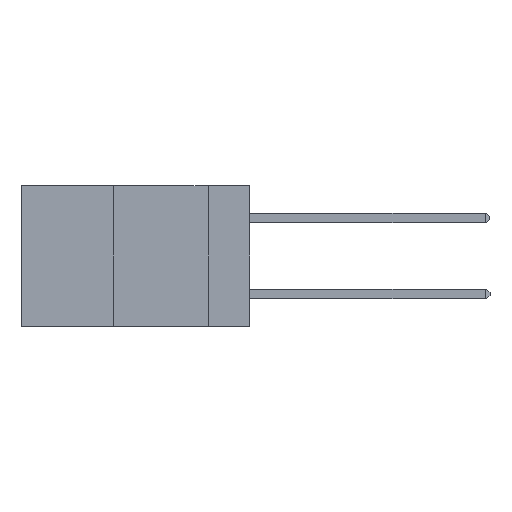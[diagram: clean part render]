
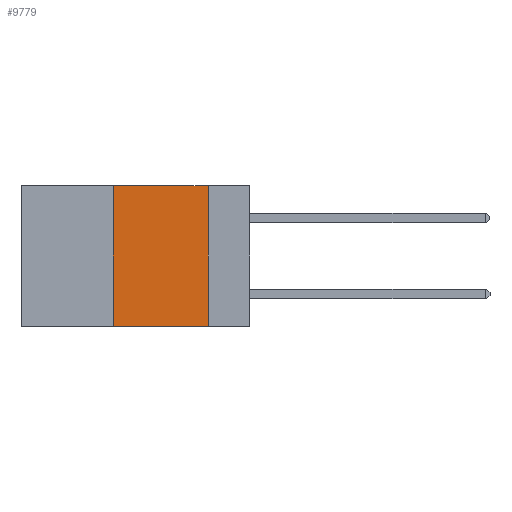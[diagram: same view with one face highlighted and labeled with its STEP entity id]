
A CAD part, left-side view. The second image highlights one B-rep face of the part: STEP entity #9779.
In plain terms, the highlighted planar face has unit normal (-1, 0, 0).
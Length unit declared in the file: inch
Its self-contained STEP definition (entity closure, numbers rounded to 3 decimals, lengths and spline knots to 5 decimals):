
#156 = CARTESIAN_POINT ( 'NONE',  ( 0., 0.6, 0. ) ) ;
#357 = DIRECTION ( 'NONE',  ( 0., 0., 1. ) ) ;
#439 = VERTEX_POINT ( 'NONE', #22396 ) ;
#813 = ORIENTED_EDGE ( 'NONE', *, *, #6139, .F. ) ;
#903 = EDGE_CURVE ( 'NONE', #3116, #18220, #6308, .T. ) ;
#1308 = CARTESIAN_POINT ( 'NONE',  ( 0., 0.6, 0. ) ) ;
#1581 = DIRECTION ( 'NONE',  ( 0., 0., -1. ) ) ;
#2209 = DIRECTION ( 'NONE',  ( 0., -1., 0. ) ) ;
#3116 = VERTEX_POINT ( 'NONE', #4890 ) ;
#4160 = DIRECTION ( 'NONE',  ( 0., -1., 0. ) ) ;
#4272 = FACE_OUTER_BOUND ( 'NONE', #5116, .T. ) ;
#4890 = CARTESIAN_POINT ( 'NONE',  ( 0., 0.36, -0.37 ) ) ;
#4979 = VECTOR ( 'NONE', #2209, 39.37008 ) ;
#5116 = EDGE_LOOP ( 'NONE', ( #8325, #813, #5667, #7925 ) ) ;
#5621 = VECTOR ( 'NONE', #1581, 39.37008 ) ;
#5667 = ORIENTED_EDGE ( 'NONE', *, *, #14387, .F. ) ;
#6139 = EDGE_CURVE ( 'NONE', #11145, #439, #9747, .T. ) ;
#6189 = LINE ( 'NONE', #10545, #5621 ) ;
#6308 = LINE ( 'NONE', #18498, #11646 ) ;
#6598 = LINE ( 'NONE', #20050, #20234 ) ;
#7240 = CARTESIAN_POINT ( 'NONE',  ( 0., 0.11, -0.37 ) ) ;
#7883 = AXIS2_PLACEMENT_3D ( 'NONE', #1308, #22674, #12191 ) ;
#7925 = ORIENTED_EDGE ( 'NONE', *, *, #903, .T. ) ;
#8325 = ORIENTED_EDGE ( 'NONE', *, *, #18668, .F. ) ;
#9747 = LINE ( 'NONE', #156, #4979 ) ;
#9779 = ADVANCED_FACE ( 'NONE', ( #4272 ), #20955, .F. ) ;
#10545 = CARTESIAN_POINT ( 'NONE',  ( 0., 0.11, 0. ) ) ;
#11145 = VERTEX_POINT ( 'NONE', #17614 ) ;
#11646 = VECTOR ( 'NONE', #4160, 39.37008 ) ;
#12191 = DIRECTION ( 'NONE',  ( 0., 0., -1. ) ) ;
#14387 = EDGE_CURVE ( 'NONE', #3116, #11145, #6598, .T. ) ;
#17614 = CARTESIAN_POINT ( 'NONE',  ( 0., 0.36, 0. ) ) ;
#18220 = VERTEX_POINT ( 'NONE', #7240 ) ;
#18498 = CARTESIAN_POINT ( 'NONE',  ( 0., 0.6, -0.37 ) ) ;
#18668 = EDGE_CURVE ( 'NONE', #439, #18220, #6189, .T. ) ;
#20050 = CARTESIAN_POINT ( 'NONE',  ( 0., 0.36, 0. ) ) ;
#20234 = VECTOR ( 'NONE', #357, 39.37008 ) ;
#20955 = PLANE ( 'NONE',  #7883 ) ;
#22396 = CARTESIAN_POINT ( 'NONE',  ( 0., 0.11, 0. ) ) ;
#22674 = DIRECTION ( 'NONE',  ( 1., 0., 0. ) ) ;
